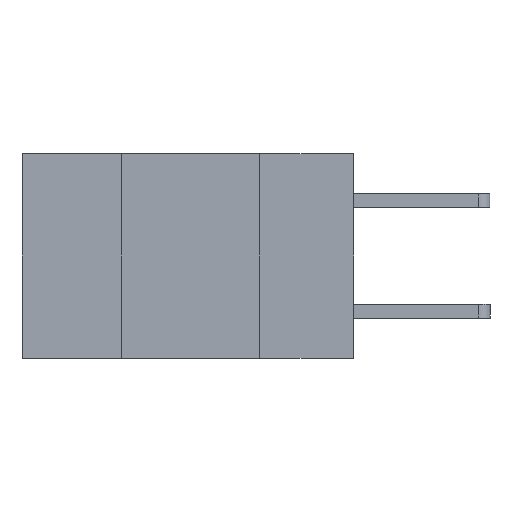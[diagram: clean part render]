
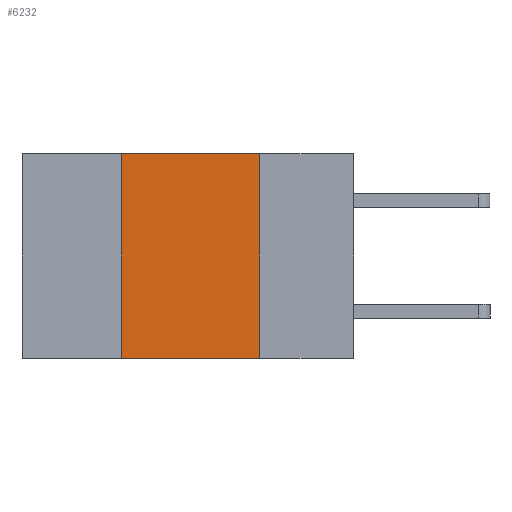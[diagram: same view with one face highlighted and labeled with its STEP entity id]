
A CAD part, left-side view. The second image highlights one B-rep face of the part: STEP entity #6232.
In plain terms, the highlighted planar face has unit normal (-1, 0, 0).
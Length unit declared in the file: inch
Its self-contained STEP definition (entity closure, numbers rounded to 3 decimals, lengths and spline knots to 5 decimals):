
#176 = AXIS2_PLACEMENT_3D ( 'NONE', #1598, #8468, #2144 ) ;
#246 = PLANE ( 'NONE',  #176 ) ;
#318 = DIRECTION ( 'NONE',  ( 0., 0., -1. ) ) ;
#419 = VECTOR ( 'NONE', #318, 39.37008 ) ;
#750 = ORIENTED_EDGE ( 'NONE', *, *, #1868, .F. ) ;
#1083 = DIRECTION ( 'NONE',  ( 0., 0., 1. ) ) ;
#1169 = CARTESIAN_POINT ( 'NONE',  ( 0., 0.42, 0. ) ) ;
#1229 = VERTEX_POINT ( 'NONE', #3282 ) ;
#1549 = EDGE_CURVE ( 'NONE', #1229, #8889, #2962, .T. ) ;
#1598 = CARTESIAN_POINT ( 'NONE',  ( 0., 0.6, 0. ) ) ;
#1868 = EDGE_CURVE ( 'NONE', #8889, #3501, #7125, .T. ) ;
#1976 = EDGE_CURVE ( 'NONE', #6032, #3501, #6529, .T. ) ;
#2072 = ORIENTED_EDGE ( 'NONE', *, *, #1549, .F. ) ;
#2144 = DIRECTION ( 'NONE',  ( 0., 0., -1. ) ) ;
#2962 = LINE ( 'NONE', #5726, #8692 ) ;
#3080 = DIRECTION ( 'NONE',  ( 0., -1., 0. ) ) ;
#3282 = CARTESIAN_POINT ( 'NONE',  ( 0., 0.42, 0. ) ) ;
#3501 = VERTEX_POINT ( 'NONE', #8269 ) ;
#3771 = EDGE_CURVE ( 'NONE', #6032, #1229, #8174, .T. ) ;
#3985 = EDGE_LOOP ( 'NONE', ( #750, #2072, #7602, #8241 ) ) ;
#5038 = CARTESIAN_POINT ( 'NONE',  ( 0., 0.6, -0.37 ) ) ;
#5345 = VECTOR ( 'NONE', #3080, 39.37008 ) ;
#5726 = CARTESIAN_POINT ( 'NONE',  ( 0., 0.6, 0. ) ) ;
#5761 = FACE_OUTER_BOUND ( 'NONE', #3985, .T. ) ;
#6032 = VERTEX_POINT ( 'NONE', #7928 ) ;
#6232 = ADVANCED_FACE ( 'NONE', ( #5761 ), #246, .F. ) ;
#6529 = LINE ( 'NONE', #5038, #5345 ) ;
#6725 = CARTESIAN_POINT ( 'NONE',  ( 0., 0.17, 0. ) ) ;
#7119 = VECTOR ( 'NONE', #1083, 39.37008 ) ;
#7125 = LINE ( 'NONE', #7172, #419 ) ;
#7172 = CARTESIAN_POINT ( 'NONE',  ( 0., 0.17, 0. ) ) ;
#7602 = ORIENTED_EDGE ( 'NONE', *, *, #3771, .F. ) ;
#7928 = CARTESIAN_POINT ( 'NONE',  ( 0., 0.42, -0.37 ) ) ;
#8174 = LINE ( 'NONE', #1169, #7119 ) ;
#8241 = ORIENTED_EDGE ( 'NONE', *, *, #1976, .T. ) ;
#8269 = CARTESIAN_POINT ( 'NONE',  ( 0., 0.17, -0.37 ) ) ;
#8468 = DIRECTION ( 'NONE',  ( 1., 0., 0. ) ) ;
#8514 = DIRECTION ( 'NONE',  ( 0., -1., 0. ) ) ;
#8692 = VECTOR ( 'NONE', #8514, 39.37008 ) ;
#8889 = VERTEX_POINT ( 'NONE', #6725 ) ;
